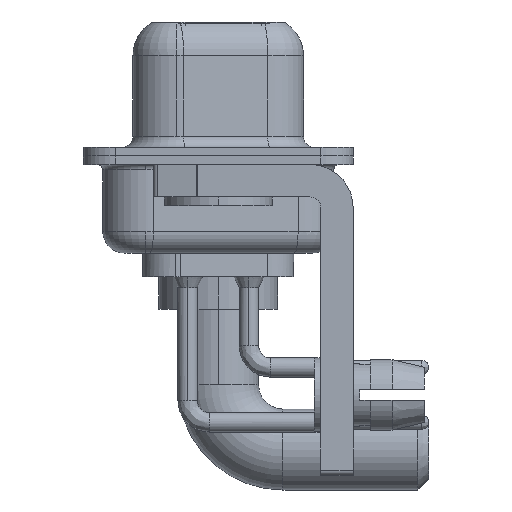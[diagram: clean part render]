
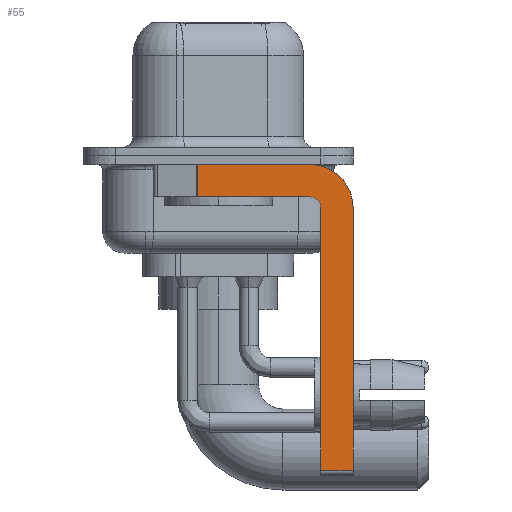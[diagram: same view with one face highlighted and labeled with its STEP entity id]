
A CAD part, left-side view. The second image highlights one B-rep face of the part: STEP entity #55.
In plain terms, the highlighted planar face has unit normal (-1, 0, 0).
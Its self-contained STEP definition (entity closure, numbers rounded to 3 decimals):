
#55 = ADVANCED_FACE ( 'NONE', ( #20921 ), #1307, .F. ) ;
#372 = VECTOR ( 'NONE', #19474, 1000. ) ;
#433 = VECTOR ( 'NONE', #6247, 1000. ) ;
#834 = DIRECTION ( 'NONE',  ( 0., -1., 0. ) ) ;
#1125 = CARTESIAN_POINT ( 'NONE',  ( -2.9, -4.75, -14.8 ) ) ;
#1307 = PLANE ( 'NONE',  #5292 ) ;
#2031 = AXIS2_PLACEMENT_3D ( 'NONE', #12521, #10829, #15931 ) ;
#2511 = VERTEX_POINT ( 'NONE', #16761 ) ;
#2677 = CARTESIAN_POINT ( 'NONE',  ( -2.9, 0.978, -0.4 ) ) ;
#2701 = DIRECTION ( 'NONE',  ( 0., 0., -1. ) ) ;
#3467 = ORIENTED_EDGE ( 'NONE', *, *, #17557, .T. ) ;
#3609 = ORIENTED_EDGE ( 'NONE', *, *, #9659, .F. ) ;
#4050 = VERTEX_POINT ( 'NONE', #9621 ) ;
#4339 = LINE ( 'NONE', #5944, #4397 ) ;
#4397 = VECTOR ( 'NONE', #12215, 1000. ) ;
#4431 = CARTESIAN_POINT ( 'NONE',  ( -2.9, -4.25, -2.4 ) ) ;
#4620 = DIRECTION ( 'NONE',  ( 1., 0., 0. ) ) ;
#5103 = CARTESIAN_POINT ( 'NONE',  ( -2.9, -4.25, -0.4 ) ) ;
#5267 = VERTEX_POINT ( 'NONE', #17525 ) ;
#5292 = AXIS2_PLACEMENT_3D ( 'NONE', #20818, #4620, #2701 ) ;
#5808 = LINE ( 'NONE', #1125, #14257 ) ;
#5841 = VERTEX_POINT ( 'NONE', #5103 ) ;
#5881 = EDGE_LOOP ( 'NONE', ( #14490, #10680, #10324, #16157, #9702, #3467, #3609, #20134 ) ) ;
#5928 = DIRECTION ( 'NONE',  ( -1., 0., 0. ) ) ;
#5944 = CARTESIAN_POINT ( 'NONE',  ( -2.9, -4.25, -14.55 ) ) ;
#6047 = DIRECTION ( 'NONE',  ( 0., 1., 0. ) ) ;
#6247 = DIRECTION ( 'NONE',  ( 0., 0., -1. ) ) ;
#7705 = EDGE_CURVE ( 'NONE', #14038, #10638, #11147, .T. ) ;
#8522 = AXIS2_PLACEMENT_3D ( 'NONE', #4431, #5928, #9550 ) ;
#8939 = CARTESIAN_POINT ( 'NONE',  ( -2.9, -6.25, -14.55 ) ) ;
#9004 = EDGE_CURVE ( 'NONE', #5267, #10638, #9265, .T. ) ;
#9265 = LINE ( 'NONE', #17344, #16079 ) ;
#9550 = DIRECTION ( 'NONE',  ( 0., 0., 1. ) ) ;
#9621 = CARTESIAN_POINT ( 'NONE',  ( -2.9, -6.25, -2.4 ) ) ;
#9659 = EDGE_CURVE ( 'NONE', #4050, #17632, #11248, .T. ) ;
#9702 = ORIENTED_EDGE ( 'NONE', *, *, #14911, .F. ) ;
#10027 = VERTEX_POINT ( 'NONE', #18535 ) ;
#10324 = ORIENTED_EDGE ( 'NONE', *, *, #9004, .F. ) ;
#10540 = EDGE_CURVE ( 'NONE', #10027, #5267, #16327, .T. ) ;
#10638 = VERTEX_POINT ( 'NONE', #17533 ) ;
#10680 = ORIENTED_EDGE ( 'NONE', *, *, #7705, .T. ) ;
#10829 = DIRECTION ( 'NONE',  ( 1., 0., 0. ) ) ;
#11147 = LINE ( 'NONE', #16253, #372 ) ;
#11248 = LINE ( 'NONE', #17846, #433 ) ;
#12215 = DIRECTION ( 'NONE',  ( 0., -1., 0. ) ) ;
#12521 = CARTESIAN_POINT ( 'NONE',  ( -2.9, -4.25, -2.4 ) ) ;
#13456 = EDGE_CURVE ( 'NONE', #14038, #5841, #15429, .T. ) ;
#13929 = CARTESIAN_POINT ( 'NONE',  ( -2.9, 3., -0.4 ) ) ;
#14038 = VERTEX_POINT ( 'NONE', #2677 ) ;
#14257 = VECTOR ( 'NONE', #20701, 1000. ) ;
#14490 = ORIENTED_EDGE ( 'NONE', *, *, #13456, .F. ) ;
#14911 = EDGE_CURVE ( 'NONE', #2511, #10027, #5808, .T. ) ;
#15429 = LINE ( 'NONE', #13929, #19800 ) ;
#15931 = DIRECTION ( 'NONE',  ( 0., 0., -1. ) ) ;
#16079 = VECTOR ( 'NONE', #6047, 1000. ) ;
#16157 = ORIENTED_EDGE ( 'NONE', *, *, #10540, .F. ) ;
#16253 = CARTESIAN_POINT ( 'NONE',  ( -2.9, 0.978, -1.9 ) ) ;
#16327 = CIRCLE ( 'NONE', #8522, 0.5 ) ;
#16761 = CARTESIAN_POINT ( 'NONE',  ( -2.9, -4.75, -14.55 ) ) ;
#17344 = CARTESIAN_POINT ( 'NONE',  ( -2.9, -4.25, -1.9 ) ) ;
#17525 = CARTESIAN_POINT ( 'NONE',  ( -2.9, -4.25, -1.9 ) ) ;
#17533 = CARTESIAN_POINT ( 'NONE',  ( -2.9, 0.978, -1.9 ) ) ;
#17557 = EDGE_CURVE ( 'NONE', #2511, #17632, #4339, .T. ) ;
#17632 = VERTEX_POINT ( 'NONE', #8939 ) ;
#17846 = CARTESIAN_POINT ( 'NONE',  ( -2.9, -6.25, -2.4 ) ) ;
#18535 = CARTESIAN_POINT ( 'NONE',  ( -2.9, -4.75, -2.4 ) ) ;
#19474 = DIRECTION ( 'NONE',  ( 0., 0., -1. ) ) ;
#19642 = EDGE_CURVE ( 'NONE', #5841, #4050, #20412, .T. ) ;
#19800 = VECTOR ( 'NONE', #834, 1000. ) ;
#20134 = ORIENTED_EDGE ( 'NONE', *, *, #19642, .F. ) ;
#20412 = CIRCLE ( 'NONE', #2031, 2. ) ;
#20701 = DIRECTION ( 'NONE',  ( 0., 0., 1. ) ) ;
#20818 = CARTESIAN_POINT ( 'NONE',  ( -2.9, -4.25, -2.4 ) ) ;
#20921 = FACE_OUTER_BOUND ( 'NONE', #5881, .T. ) ;
